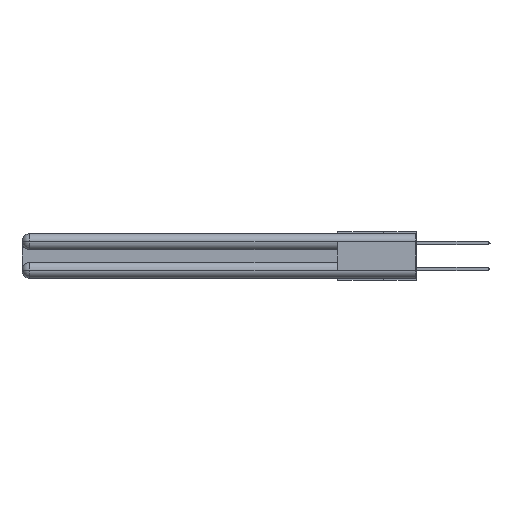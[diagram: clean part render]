
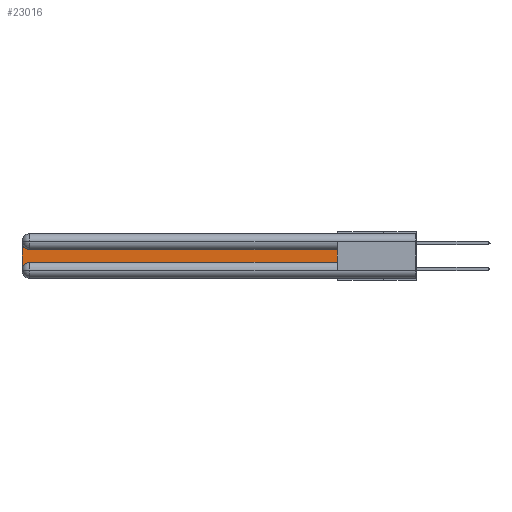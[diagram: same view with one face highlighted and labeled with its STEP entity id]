
A CAD part, left-side view. The second image highlights one B-rep face of the part: STEP entity #23016.
In plain terms, the highlighted planar face has unit normal (-1, 0, 0).
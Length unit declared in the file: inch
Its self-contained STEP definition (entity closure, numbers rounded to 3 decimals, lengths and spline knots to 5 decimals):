
#243 = ORIENTED_EDGE ( 'NONE', *, *, #12745, .T. ) ;
#549 = EDGE_CURVE ( 'NONE', #12064, #24664, #13657, .T. ) ;
#746 = VECTOR ( 'NONE', #8390, 39.37008 ) ;
#1863 = CARTESIAN_POINT ( 'NONE',  ( 0.075, 3., -0.2775 ) ) ;
#2495 = CARTESIAN_POINT ( 'NONE',  ( 0.075, 2.94, -0.1225 ) ) ;
#2992 = VERTEX_POINT ( 'NONE', #8751 ) ;
#3032 = LINE ( 'NONE', #10473, #746 ) ;
#3545 = EDGE_CURVE ( 'NONE', #24664, #21677, #3032, .T. ) ;
#4138 = DIRECTION ( 'NONE',  ( 0., 0., -1. ) ) ;
#4345 = VECTOR ( 'NONE', #19691, 39.37008 ) ;
#5185 = AXIS2_PLACEMENT_3D ( 'NONE', #24997, #10798, #15593 ) ;
#5266 = AXIS2_PLACEMENT_3D ( 'NONE', #5586, #22519, #15351 ) ;
#5586 = CARTESIAN_POINT ( 'NONE',  ( 0.075, 2.94, -0.0625 ) ) ;
#5644 = EDGE_CURVE ( 'NONE', #2992, #12064, #6205, .T. ) ;
#5725 = VERTEX_POINT ( 'NONE', #11350 ) ;
#6205 = LINE ( 'NONE', #20519, #28099 ) ;
#7542 = LINE ( 'NONE', #21676, #27602 ) ;
#8390 = DIRECTION ( 'NONE',  ( 0., -1., 0. ) ) ;
#8410 = PLANE ( 'NONE',  #5185 ) ;
#8751 = CARTESIAN_POINT ( 'NONE',  ( 0.075, 3., -0.0625 ) ) ;
#9038 = DIRECTION ( 'NONE',  ( 1., 0., 0. ) ) ;
#9265 = VERTEX_POINT ( 'NONE', #2495 ) ;
#10473 = CARTESIAN_POINT ( 'NONE',  ( 0.075, 0.6, -0.2175 ) ) ;
#10610 = FACE_OUTER_BOUND ( 'NONE', #15947, .T. ) ;
#10798 = DIRECTION ( 'NONE',  ( 1., 0., 0. ) ) ;
#11028 = EDGE_CURVE ( 'NONE', #21677, #5725, #7542, .T. ) ;
#11350 = CARTESIAN_POINT ( 'NONE',  ( 0.075, 0.6, -0.1225 ) ) ;
#12064 = VERTEX_POINT ( 'NONE', #1863 ) ;
#12745 = EDGE_CURVE ( 'NONE', #5725, #9265, #18513, .T. ) ;
#12848 = CARTESIAN_POINT ( 'NONE',  ( 0.075, 2.94, -0.2775 ) ) ;
#13657 = CIRCLE ( 'NONE', #19068, 0.06 ) ;
#14970 = CARTESIAN_POINT ( 'NONE',  ( 0.075, 2.94, -0.2175 ) ) ;
#15351 = DIRECTION ( 'NONE',  ( 0., 0., -1. ) ) ;
#15593 = DIRECTION ( 'NONE',  ( 0., 0., -1. ) ) ;
#15947 = EDGE_LOOP ( 'NONE', ( #243, #22267, #23904, #15990, #21370, #20246 ) ) ;
#15990 = ORIENTED_EDGE ( 'NONE', *, *, #549, .T. ) ;
#16814 = EDGE_CURVE ( 'NONE', #9265, #2992, #29887, .T. ) ;
#18513 = LINE ( 'NONE', #26700, #4345 ) ;
#19068 = AXIS2_PLACEMENT_3D ( 'NONE', #12848, #9038, #4138 ) ;
#19691 = DIRECTION ( 'NONE',  ( 0., 1., 0. ) ) ;
#20246 = ORIENTED_EDGE ( 'NONE', *, *, #11028, .T. ) ;
#20318 = DIRECTION ( 'NONE',  ( 0., 0., -1. ) ) ;
#20519 = CARTESIAN_POINT ( 'NONE',  ( 0.075, 3., -0.2175 ) ) ;
#21370 = ORIENTED_EDGE ( 'NONE', *, *, #3545, .T. ) ;
#21676 = CARTESIAN_POINT ( 'NONE',  ( 0.075, 0.6, -0.2175 ) ) ;
#21677 = VERTEX_POINT ( 'NONE', #26623 ) ;
#22267 = ORIENTED_EDGE ( 'NONE', *, *, #16814, .T. ) ;
#22519 = DIRECTION ( 'NONE',  ( 1., 0., 0. ) ) ;
#23016 = ADVANCED_FACE ( 'NONE', ( #10610 ), #8410, .F. ) ;
#23904 = ORIENTED_EDGE ( 'NONE', *, *, #5644, .T. ) ;
#24664 = VERTEX_POINT ( 'NONE', #14970 ) ;
#24997 = CARTESIAN_POINT ( 'NONE',  ( 0.075, 3., -0.1225 ) ) ;
#26521 = DIRECTION ( 'NONE',  ( 0., 0., 1. ) ) ;
#26623 = CARTESIAN_POINT ( 'NONE',  ( 0.075, 0.6, -0.2175 ) ) ;
#26700 = CARTESIAN_POINT ( 'NONE',  ( 0.075, 0.6, -0.1225 ) ) ;
#27602 = VECTOR ( 'NONE', #26521, 39.37008 ) ;
#28099 = VECTOR ( 'NONE', #20318, 39.37008 ) ;
#29887 = CIRCLE ( 'NONE', #5266, 0.06 ) ;
